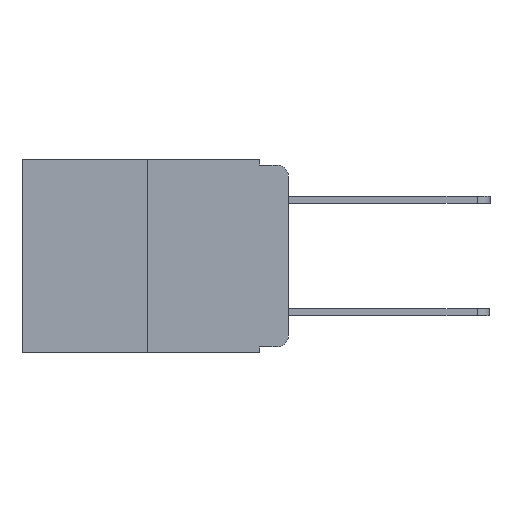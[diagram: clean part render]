
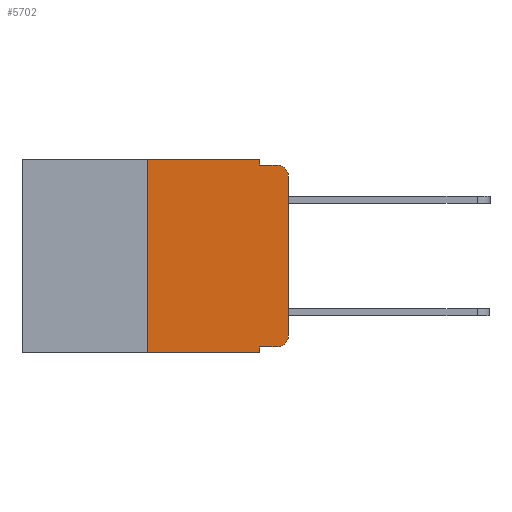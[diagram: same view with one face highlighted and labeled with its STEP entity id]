
A CAD part, left-side view. The second image highlights one B-rep face of the part: STEP entity #5702.
In plain terms, the highlighted planar face has unit normal (-1, 0, 0).
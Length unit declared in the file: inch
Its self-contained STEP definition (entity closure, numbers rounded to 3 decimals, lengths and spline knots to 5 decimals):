
#216 = ORIENTED_EDGE ( 'NONE', *, *, #3015, .F. ) ;
#377 = DIRECTION ( 'NONE',  ( 0., -1., 0. ) ) ;
#480 = LINE ( 'NONE', #12808, #14556 ) ;
#995 = VECTOR ( 'NONE', #1513, 39.37008 ) ;
#1205 = ORIENTED_EDGE ( 'NONE', *, *, #11242, .T. ) ;
#1513 = DIRECTION ( 'NONE',  ( 0., 0., 1. ) ) ;
#1612 = DIRECTION ( 'NONE',  ( 1., 0., 0. ) ) ;
#2063 = LINE ( 'NONE', #12429, #12939 ) ;
#2183 = EDGE_CURVE ( 'NONE', #8609, #10589, #7985, .T. ) ;
#2215 = DIRECTION ( 'NONE',  ( 0., 0., -1. ) ) ;
#2632 = ORIENTED_EDGE ( 'NONE', *, *, #9234, .F. ) ;
#2722 = VERTEX_POINT ( 'NONE', #13137 ) ;
#2816 = VECTOR ( 'NONE', #7267, 39.37008 ) ;
#2832 = ORIENTED_EDGE ( 'NONE', *, *, #11410, .T. ) ;
#2870 = EDGE_CURVE ( 'NONE', #8987, #16979, #17124, .T. ) ;
#2878 = CARTESIAN_POINT ( 'NONE',  ( 0., 0.02, -0.03 ) ) ;
#2991 = CARTESIAN_POINT ( 'NONE',  ( 0., 0., 0. ) ) ;
#3015 = EDGE_CURVE ( 'NONE', #2722, #4468, #8396, .T. ) ;
#3017 = VERTEX_POINT ( 'NONE', #11347 ) ;
#3845 = DIRECTION ( 'NONE',  ( 0., 0., -1. ) ) ;
#4240 = FACE_OUTER_BOUND ( 'NONE', #9815, .T. ) ;
#4468 = VERTEX_POINT ( 'NONE', #16594 ) ;
#4681 = VECTOR ( 'NONE', #3845, 39.37008 ) ;
#5187 = CARTESIAN_POINT ( 'NONE',  ( 0., 0.02, -0.333 ) ) ;
#5432 = DIRECTION ( 'NONE',  ( -1., 0., 0. ) ) ;
#5702 = ADVANCED_FACE ( 'NONE', ( #4240 ), #16016, .F. ) ;
#5777 = CARTESIAN_POINT ( 'NONE',  ( 0., 0.25, -0.343 ) ) ;
#6069 = CARTESIAN_POINT ( 'NONE',  ( 0., 0.02, -0.01 ) ) ;
#6266 = CARTESIAN_POINT ( 'NONE',  ( 0., 0.051, -0.333 ) ) ;
#6306 = DIRECTION ( 'NONE',  ( 0., -1., 0. ) ) ;
#6342 = ORIENTED_EDGE ( 'NONE', *, *, #2183, .T. ) ;
#6551 = ORIENTED_EDGE ( 'NONE', *, *, #14034, .F. ) ;
#7091 = CARTESIAN_POINT ( 'NONE',  ( 0., 0.051, -0.343 ) ) ;
#7267 = DIRECTION ( 'NONE',  ( 0., -1., 0. ) ) ;
#7395 = VECTOR ( 'NONE', #6306, 39.37008 ) ;
#7697 = LINE ( 'NONE', #2991, #995 ) ;
#7859 = CARTESIAN_POINT ( 'NONE',  ( 0., 0.051, 0. ) ) ;
#7871 = EDGE_CURVE ( 'NONE', #8436, #11172, #11191, .T. ) ;
#7985 = CIRCLE ( 'NONE', #8141, 0.02 ) ;
#8073 = ORIENTED_EDGE ( 'NONE', *, *, #13843, .F. ) ;
#8122 = VECTOR ( 'NONE', #2215, 39.37008 ) ;
#8141 = AXIS2_PLACEMENT_3D ( 'NONE', #12531, #5432, #8718 ) ;
#8396 = LINE ( 'NONE', #7859, #4681 ) ;
#8436 = VERTEX_POINT ( 'NONE', #6266 ) ;
#8609 = VERTEX_POINT ( 'NONE', #5187 ) ;
#8628 = CARTESIAN_POINT ( 'NONE',  ( 0., 0., -0.03 ) ) ;
#8718 = DIRECTION ( 'NONE',  ( 0., 0., -1. ) ) ;
#8863 = ORIENTED_EDGE ( 'NONE', *, *, #2870, .T. ) ;
#8987 = VERTEX_POINT ( 'NONE', #8628 ) ;
#9217 = CARTESIAN_POINT ( 'NONE',  ( 0., 0.051, 0. ) ) ;
#9234 = EDGE_CURVE ( 'NONE', #4468, #16979, #10948, .T. ) ;
#9311 = VECTOR ( 'NONE', #377, 39.37008 ) ;
#9313 = ORIENTED_EDGE ( 'NONE', *, *, #10419, .T. ) ;
#9815 = EDGE_LOOP ( 'NONE', ( #9313, #8863, #2632, #216, #6551, #8073, #1205, #14168, #2832, #6342 ) ) ;
#9896 = DIRECTION ( 'NONE',  ( 0., 0., 1. ) ) ;
#10419 = EDGE_CURVE ( 'NONE', #10589, #8987, #7697, .T. ) ;
#10589 = VERTEX_POINT ( 'NONE', #12763 ) ;
#10948 = LINE ( 'NONE', #11607, #7395 ) ;
#11123 = DIRECTION ( 'NONE',  ( 0., 0., -1. ) ) ;
#11172 = VERTEX_POINT ( 'NONE', #7091 ) ;
#11191 = LINE ( 'NONE', #9217, #8122 ) ;
#11219 = DIRECTION ( 'NONE',  ( -1., 0., 0. ) ) ;
#11242 = EDGE_CURVE ( 'NONE', #11924, #11172, #13985, .T. ) ;
#11274 = DIRECTION ( 'NONE',  ( 0., 0., -1. ) ) ;
#11347 = CARTESIAN_POINT ( 'NONE',  ( 0., 0.25, 0. ) ) ;
#11410 = EDGE_CURVE ( 'NONE', #8436, #8609, #480, .T. ) ;
#11607 = CARTESIAN_POINT ( 'NONE',  ( 0., 0.051, -0.01 ) ) ;
#11924 = VERTEX_POINT ( 'NONE', #5777 ) ;
#12407 = AXIS2_PLACEMENT_3D ( 'NONE', #2878, #11219, #11123 ) ;
#12429 = CARTESIAN_POINT ( 'NONE',  ( 0., 0.25, 0. ) ) ;
#12531 = CARTESIAN_POINT ( 'NONE',  ( 0., 0.02, -0.313 ) ) ;
#12757 = CARTESIAN_POINT ( 'NONE',  ( 0., 0.473, 0. ) ) ;
#12763 = CARTESIAN_POINT ( 'NONE',  ( 0., 0., -0.313 ) ) ;
#12808 = CARTESIAN_POINT ( 'NONE',  ( 0., 0.051, -0.333 ) ) ;
#12939 = VECTOR ( 'NONE', #9896, 39.37008 ) ;
#13137 = CARTESIAN_POINT ( 'NONE',  ( 0., 0.051, 0. ) ) ;
#13843 = EDGE_CURVE ( 'NONE', #11924, #3017, #2063, .T. ) ;
#13985 = LINE ( 'NONE', #16221, #2816 ) ;
#14034 = EDGE_CURVE ( 'NONE', #3017, #2722, #16027, .T. ) ;
#14168 = ORIENTED_EDGE ( 'NONE', *, *, #7871, .F. ) ;
#14556 = VECTOR ( 'NONE', #15313, 39.37008 ) ;
#15313 = DIRECTION ( 'NONE',  ( 0., -1., 0. ) ) ;
#16016 = PLANE ( 'NONE',  #17030 ) ;
#16027 = LINE ( 'NONE', #12757, #9311 ) ;
#16221 = CARTESIAN_POINT ( 'NONE',  ( 0., 0.473, -0.343 ) ) ;
#16319 = CARTESIAN_POINT ( 'NONE',  ( 0., 0.473, 0. ) ) ;
#16594 = CARTESIAN_POINT ( 'NONE',  ( 0., 0.051, -0.01 ) ) ;
#16979 = VERTEX_POINT ( 'NONE', #6069 ) ;
#17030 = AXIS2_PLACEMENT_3D ( 'NONE', #16319, #1612, #11274 ) ;
#17124 = CIRCLE ( 'NONE', #12407, 0.02 ) ;
